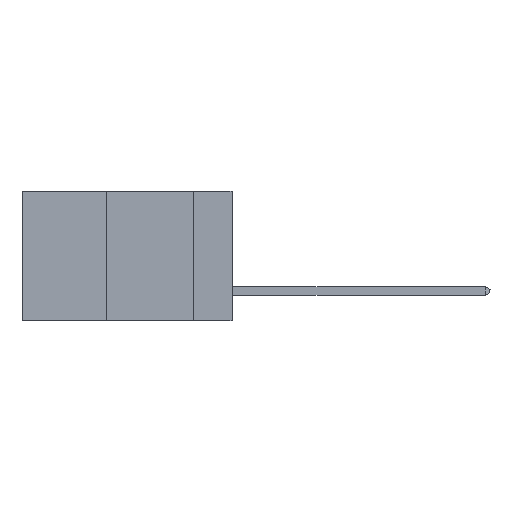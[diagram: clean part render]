
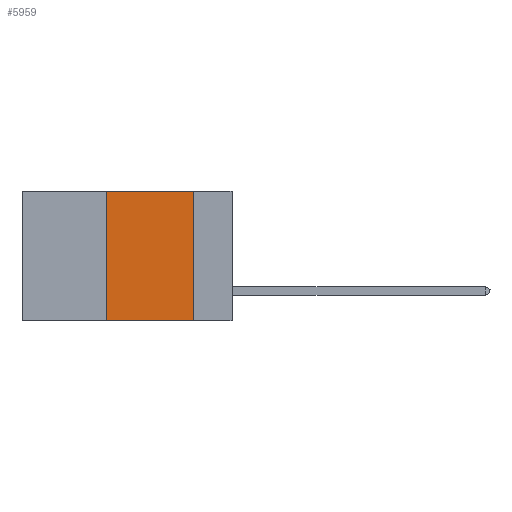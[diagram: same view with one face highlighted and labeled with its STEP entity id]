
A CAD part, left-side view. The second image highlights one B-rep face of the part: STEP entity #5959.
In plain terms, the highlighted planar face has unit normal (-1, 0, 0).
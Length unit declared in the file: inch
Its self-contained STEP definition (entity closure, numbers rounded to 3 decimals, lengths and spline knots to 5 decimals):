
#368 = DIRECTION ( 'NONE',  ( 0., -1., 0. ) ) ;
#731 = LINE ( 'NONE', #9965, #34366 ) ;
#934 = CARTESIAN_POINT ( 'NONE',  ( 0., 0.36, -0.37 ) ) ;
#2512 = VECTOR ( 'NONE', #40422, 39.37008 ) ;
#4912 = LINE ( 'NONE', #21861, #7882 ) ;
#5959 = ADVANCED_FACE ( 'NONE', ( #35973 ), #11257, .F. ) ;
#7882 = VECTOR ( 'NONE', #21731, 39.37008 ) ;
#8546 = EDGE_CURVE ( 'NONE', #18600, #30034, #22992, .T. ) ;
#8792 = ORIENTED_EDGE ( 'NONE', *, *, #37082, .F. ) ;
#9965 = CARTESIAN_POINT ( 'NONE',  ( 0., 0.6, -0.37 ) ) ;
#11257 = PLANE ( 'NONE',  #33826 ) ;
#13861 = CARTESIAN_POINT ( 'NONE',  ( 0., 0.36, 0. ) ) ;
#14362 = VECTOR ( 'NONE', #368, 39.37008 ) ;
#16682 = CARTESIAN_POINT ( 'NONE',  ( 0., 0.6, 0. ) ) ;
#18600 = VERTEX_POINT ( 'NONE', #29082 ) ;
#18734 = LINE ( 'NONE', #13861, #2512 ) ;
#20734 = VERTEX_POINT ( 'NONE', #36545 ) ;
#20955 = ORIENTED_EDGE ( 'NONE', *, *, #8546, .F. ) ;
#21731 = DIRECTION ( 'NONE',  ( 0., 0., -1. ) ) ;
#21861 = CARTESIAN_POINT ( 'NONE',  ( 0., 0.11, 0. ) ) ;
#22992 = LINE ( 'NONE', #16682, #14362 ) ;
#24462 = DIRECTION ( 'NONE',  ( 1., 0., 0. ) ) ;
#24612 = CARTESIAN_POINT ( 'NONE',  ( 0., 0.6, 0. ) ) ;
#26272 = VERTEX_POINT ( 'NONE', #934 ) ;
#27559 = EDGE_CURVE ( 'NONE', #26272, #18600, #18734, .T. ) ;
#29082 = CARTESIAN_POINT ( 'NONE',  ( 0., 0.36, 0. ) ) ;
#30034 = VERTEX_POINT ( 'NONE', #30069 ) ;
#30069 = CARTESIAN_POINT ( 'NONE',  ( 0., 0.11, 0. ) ) ;
#31603 = ORIENTED_EDGE ( 'NONE', *, *, #37404, .T. ) ;
#32676 = ORIENTED_EDGE ( 'NONE', *, *, #27559, .F. ) ;
#33826 = AXIS2_PLACEMENT_3D ( 'NONE', #24612, #24462, #34059 ) ;
#34059 = DIRECTION ( 'NONE',  ( 0., 0., -1. ) ) ;
#34366 = VECTOR ( 'NONE', #35619, 39.37008 ) ;
#35619 = DIRECTION ( 'NONE',  ( 0., -1., 0. ) ) ;
#35893 = EDGE_LOOP ( 'NONE', ( #8792, #20955, #32676, #31603 ) ) ;
#35973 = FACE_OUTER_BOUND ( 'NONE', #35893, .T. ) ;
#36545 = CARTESIAN_POINT ( 'NONE',  ( 0., 0.11, -0.37 ) ) ;
#37082 = EDGE_CURVE ( 'NONE', #30034, #20734, #4912, .T. ) ;
#37404 = EDGE_CURVE ( 'NONE', #26272, #20734, #731, .T. ) ;
#40422 = DIRECTION ( 'NONE',  ( 0., 0., 1. ) ) ;
